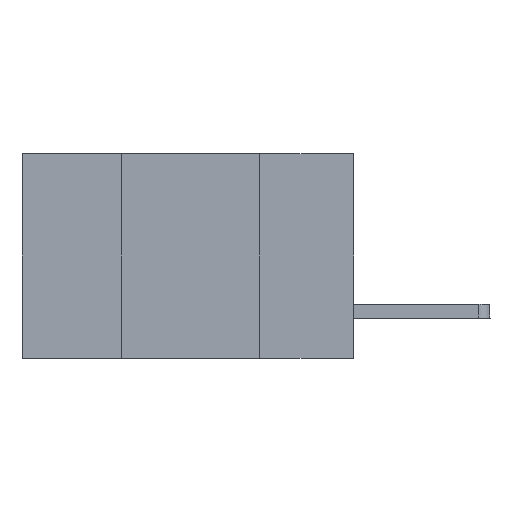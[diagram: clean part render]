
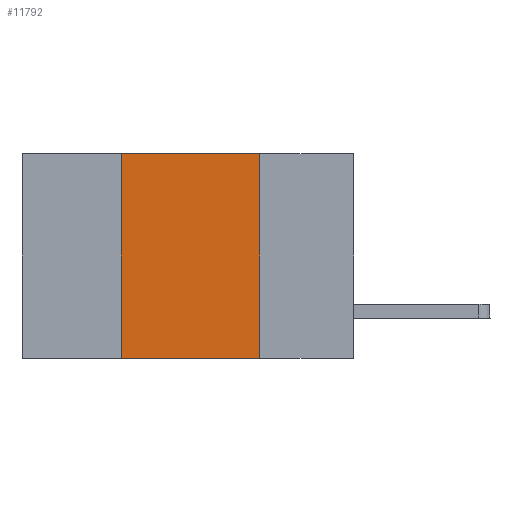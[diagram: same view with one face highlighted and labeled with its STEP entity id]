
A CAD part, left-side view. The second image highlights one B-rep face of the part: STEP entity #11792.
In plain terms, the highlighted planar face has unit normal (-1, 0, 0).
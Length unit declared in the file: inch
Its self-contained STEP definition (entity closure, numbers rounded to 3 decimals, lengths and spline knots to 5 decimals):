
#775 = EDGE_CURVE ( 'NONE', #7250, #6556, #10041, .T. ) ;
#1008 = DIRECTION ( 'NONE',  ( 0., 0., -1. ) ) ;
#1178 = CARTESIAN_POINT ( 'NONE',  ( 0., 0.6, -0.37 ) ) ;
#1180 = VERTEX_POINT ( 'NONE', #13343 ) ;
#1192 = CARTESIAN_POINT ( 'NONE',  ( 0., 0.17, -0.37 ) ) ;
#1238 = CARTESIAN_POINT ( 'NONE',  ( 0., 0.42, 0. ) ) ;
#1971 = AXIS2_PLACEMENT_3D ( 'NONE', #5125, #4239, #1008 ) ;
#2183 = LINE ( 'NONE', #6581, #4190 ) ;
#2382 = VERTEX_POINT ( 'NONE', #3786 ) ;
#3786 = CARTESIAN_POINT ( 'NONE',  ( 0., 0.42, 0. ) ) ;
#4190 = VECTOR ( 'NONE', #4527, 39.37008 ) ;
#4239 = DIRECTION ( 'NONE',  ( 1., 0., 0. ) ) ;
#4255 = ORIENTED_EDGE ( 'NONE', *, *, #12990, .F. ) ;
#4527 = DIRECTION ( 'NONE',  ( 0., -1., 0. ) ) ;
#4558 = VECTOR ( 'NONE', #7373, 39.37008 ) ;
#4685 = FACE_OUTER_BOUND ( 'NONE', #12104, .T. ) ;
#4982 = VECTOR ( 'NONE', #8809, 39.37008 ) ;
#5125 = CARTESIAN_POINT ( 'NONE',  ( 0., 0.6, 0. ) ) ;
#5498 = VECTOR ( 'NONE', #9739, 39.37008 ) ;
#5888 = PLANE ( 'NONE',  #1971 ) ;
#6556 = VERTEX_POINT ( 'NONE', #1192 ) ;
#6581 = CARTESIAN_POINT ( 'NONE',  ( 0., 0.6, 0. ) ) ;
#7250 = VERTEX_POINT ( 'NONE', #9657 ) ;
#7373 = DIRECTION ( 'NONE',  ( 0., -1., 0. ) ) ;
#8003 = LINE ( 'NONE', #1238, #5498 ) ;
#8656 = ORIENTED_EDGE ( 'NONE', *, *, #11701, .F. ) ;
#8809 = DIRECTION ( 'NONE',  ( 0., 0., -1. ) ) ;
#9657 = CARTESIAN_POINT ( 'NONE',  ( 0., 0.42, -0.37 ) ) ;
#9739 = DIRECTION ( 'NONE',  ( 0., 0., 1. ) ) ;
#10041 = LINE ( 'NONE', #1178, #4558 ) ;
#10116 = LINE ( 'NONE', #12938, #4982 ) ;
#10385 = ORIENTED_EDGE ( 'NONE', *, *, #775, .T. ) ;
#11701 = EDGE_CURVE ( 'NONE', #2382, #1180, #2183, .T. ) ;
#11792 = ADVANCED_FACE ( 'NONE', ( #4685 ), #5888, .F. ) ;
#12104 = EDGE_LOOP ( 'NONE', ( #4255, #8656, #13685, #10385 ) ) ;
#12938 = CARTESIAN_POINT ( 'NONE',  ( 0., 0.17, 0. ) ) ;
#12990 = EDGE_CURVE ( 'NONE', #1180, #6556, #10116, .T. ) ;
#13343 = CARTESIAN_POINT ( 'NONE',  ( 0., 0.17, 0. ) ) ;
#13399 = EDGE_CURVE ( 'NONE', #7250, #2382, #8003, .T. ) ;
#13685 = ORIENTED_EDGE ( 'NONE', *, *, #13399, .F. ) ;
